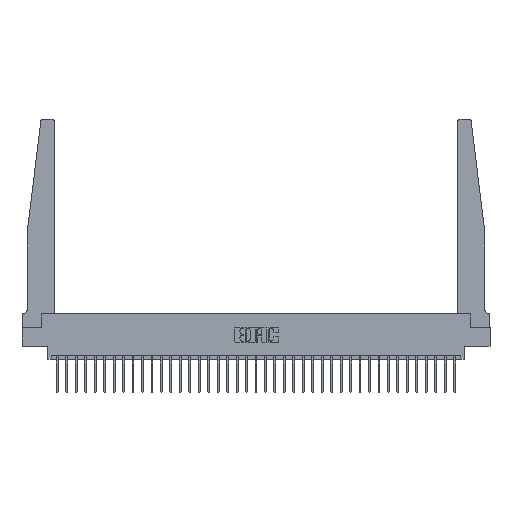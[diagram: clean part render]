
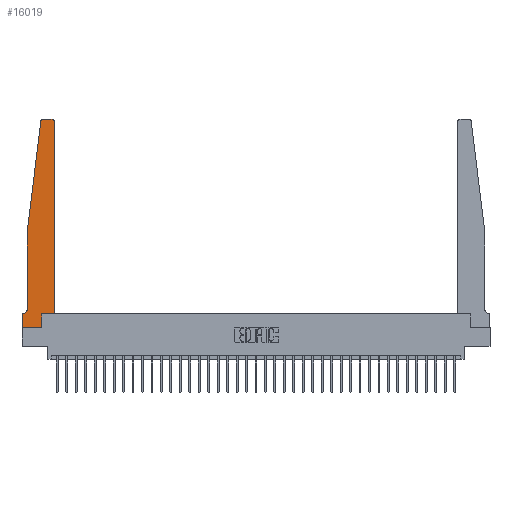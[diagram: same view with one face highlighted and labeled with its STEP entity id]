
A CAD part, top view. The second image highlights one B-rep face of the part: STEP entity #16019.
In plain terms, the highlighted planar face has unit normal (0, 0, 1).
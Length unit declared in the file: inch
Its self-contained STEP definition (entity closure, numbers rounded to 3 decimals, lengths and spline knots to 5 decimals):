
#213 = VECTOR ( 'NONE', #19562, 39.37008 ) ;
#295 = AXIS2_PLACEMENT_3D ( 'NONE', #20540, #5225, #23086 ) ;
#1039 = ORIENTED_EDGE ( 'NONE', *, *, #8763, .T. ) ;
#1201 = DIRECTION ( 'NONE',  ( -1., 0., 0. ) ) ;
#1218 = CARTESIAN_POINT ( 'NONE',  ( 0.065, 1.25, 0.37 ) ) ;
#1359 = CARTESIAN_POINT ( 'NONE',  ( 0., 0., 0.37 ) ) ;
#1548 = VERTEX_POINT ( 'NONE', #15103 ) ;
#1581 = ORIENTED_EDGE ( 'NONE', *, *, #18821, .T. ) ;
#1651 = CARTESIAN_POINT ( 'NONE',  ( 0.2605, 0.18, 0.37 ) ) ;
#1680 = VERTEX_POINT ( 'NONE', #15545 ) ;
#1836 = DIRECTION ( 'NONE',  ( 1., 0., 0. ) ) ;
#2565 = VERTEX_POINT ( 'NONE', #21839 ) ;
#2676 = LINE ( 'NONE', #16550, #31295 ) ;
#3178 = EDGE_CURVE ( 'NONE', #5346, #8923, #9283, .T. ) ;
#4044 = CARTESIAN_POINT ( 'NONE',  ( 0., 0., 0.37 ) ) ;
#4154 = DIRECTION ( 'NONE',  ( 0., -1., 0. ) ) ;
#4301 = CIRCLE ( 'NONE', #295, 0.05 ) ;
#4777 = DIRECTION ( 'NONE',  ( 0., -1., 0. ) ) ;
#4904 = AXIS2_PLACEMENT_3D ( 'NONE', #11142, #28911, #13719 ) ;
#5198 = LINE ( 'NONE', #8431, #18011 ) ;
#5225 = DIRECTION ( 'NONE',  ( 0., 0., -1. ) ) ;
#5346 = VERTEX_POINT ( 'NONE', #24933 ) ;
#5541 = CARTESIAN_POINT ( 'NONE',  ( 0.27653, 2.72, 0.37 ) ) ;
#5909 = CARTESIAN_POINT ( 'NONE',  ( 0.395, 2.72, 0.37 ) ) ;
#5992 = PLANE ( 'NONE',  #4904 ) ;
#6184 = EDGE_CURVE ( 'NONE', #6297, #2565, #2676, .T. ) ;
#6297 = VERTEX_POINT ( 'NONE', #26972 ) ;
#6372 = ORIENTED_EDGE ( 'NONE', *, *, #26674, .T. ) ;
#6871 = CARTESIAN_POINT ( 'NONE',  ( 0.425, 0.18, 0.37 ) ) ;
#7365 = LINE ( 'NONE', #25215, #20162 ) ;
#7714 = EDGE_CURVE ( 'NONE', #30909, #18710, #8582, .T. ) ;
#8124 = DIRECTION ( 'NONE',  ( 1., 0., 0. ) ) ;
#8431 = CARTESIAN_POINT ( 'NONE',  ( 0.065, 0.1875, 0.37 ) ) ;
#8477 = DIRECTION ( 'NONE',  ( 1., 0., 0. ) ) ;
#8582 = LINE ( 'NONE', #22020, #28882 ) ;
#8763 = EDGE_CURVE ( 'NONE', #2565, #27652, #12119, .T. ) ;
#8913 = EDGE_LOOP ( 'NONE', ( #11720, #1039, #6372, #1581, #9547, #12216, #17076, #16816, #17228, #18980, #19419, #20133 ) ) ;
#8923 = VERTEX_POINT ( 'NONE', #1359 ) ;
#9283 = LINE ( 'NONE', #4044, #28784 ) ;
#9547 = ORIENTED_EDGE ( 'NONE', *, *, #22452, .T. ) ;
#10999 = AXIS2_PLACEMENT_3D ( 'NONE', #5541, #23408, #8124 ) ;
#11142 = CARTESIAN_POINT ( 'NONE',  ( 0., 0.1875, 0.37 ) ) ;
#11720 = ORIENTED_EDGE ( 'NONE', *, *, #6184, .T. ) ;
#11941 = CARTESIAN_POINT ( 'NONE',  ( 0.425, 0.18, 0.37 ) ) ;
#12119 = CIRCLE ( 'NONE', #10999, 0.03 ) ;
#12216 = ORIENTED_EDGE ( 'NONE', *, *, #26487, .T. ) ;
#13167 = EDGE_CURVE ( 'NONE', #8923, #23413, #18066, .T. ) ;
#13215 = LINE ( 'NONE', #32011, #19977 ) ;
#13719 = DIRECTION ( 'NONE',  ( 1., 0., 0. ) ) ;
#14619 = CARTESIAN_POINT ( 'NONE',  ( 0., 0., 0.37 ) ) ;
#15103 = CARTESIAN_POINT ( 'NONE',  ( 0.065, 0.2375, 0.37 ) ) ;
#15545 = CARTESIAN_POINT ( 'NONE',  ( 0.425, 2.72, 0.37 ) ) ;
#16019 = ADVANCED_FACE ( 'NONE', ( #17477 ), #5992, .T. ) ;
#16267 = EDGE_CURVE ( 'NONE', #18710, #1680, #23837, .T. ) ;
#16524 = CARTESIAN_POINT ( 'NONE',  ( 0.2605, 0.18, 0.37 ) ) ;
#16550 = CARTESIAN_POINT ( 'NONE',  ( 0.25, 2.75, 0.37 ) ) ;
#16816 = ORIENTED_EDGE ( 'NONE', *, *, #13167, .T. ) ;
#16880 = EDGE_CURVE ( 'NONE', #23413, #30909, #19827, .T. ) ;
#16916 = DIRECTION ( 'NONE',  ( -0.122, -0.992, 0. ) ) ;
#17058 = VECTOR ( 'NONE', #32218, 39.37008 ) ;
#17076 = ORIENTED_EDGE ( 'NONE', *, *, #3178, .T. ) ;
#17228 = ORIENTED_EDGE ( 'NONE', *, *, #16880, .T. ) ;
#17328 = EDGE_CURVE ( 'NONE', #1680, #6297, #28116, .T. ) ;
#17477 = FACE_OUTER_BOUND ( 'NONE', #8913, .T. ) ;
#18011 = VECTOR ( 'NONE', #31153, 39.37008 ) ;
#18066 = LINE ( 'NONE', #14619, #23231 ) ;
#18710 = VERTEX_POINT ( 'NONE', #11941 ) ;
#18821 = EDGE_CURVE ( 'NONE', #19816, #1548, #7365, .T. ) ;
#18980 = ORIENTED_EDGE ( 'NONE', *, *, #7714, .T. ) ;
#19419 = ORIENTED_EDGE ( 'NONE', *, *, #16267, .T. ) ;
#19562 = DIRECTION ( 'NONE',  ( 0., 1., 0. ) ) ;
#19816 = VERTEX_POINT ( 'NONE', #1218 ) ;
#19827 = LINE ( 'NONE', #1651, #213 ) ;
#19977 = VECTOR ( 'NONE', #16916, 39.37008 ) ;
#20133 = ORIENTED_EDGE ( 'NONE', *, *, #17328, .T. ) ;
#20162 = VECTOR ( 'NONE', #4777, 39.37008 ) ;
#20540 = CARTESIAN_POINT ( 'NONE',  ( 0.015, 0.2375, 0.37 ) ) ;
#21839 = CARTESIAN_POINT ( 'NONE',  ( 0.27653, 2.75, 0.37 ) ) ;
#22020 = CARTESIAN_POINT ( 'NONE',  ( 0.425, 0.18, 0.37 ) ) ;
#22452 = EDGE_CURVE ( 'NONE', #1548, #24305, #4301, .T. ) ;
#23086 = DIRECTION ( 'NONE',  ( -1., 0., 0. ) ) ;
#23231 = VECTOR ( 'NONE', #1836, 39.37008 ) ;
#23408 = DIRECTION ( 'NONE',  ( 0., 0., 1. ) ) ;
#23413 = VERTEX_POINT ( 'NONE', #24577 ) ;
#23766 = DIRECTION ( 'NONE',  ( 0., 0., 1. ) ) ;
#23837 = LINE ( 'NONE', #6871, #17058 ) ;
#24289 = CARTESIAN_POINT ( 'NONE',  ( 0.015, 0.1875, 0.37 ) ) ;
#24305 = VERTEX_POINT ( 'NONE', #24289 ) ;
#24577 = CARTESIAN_POINT ( 'NONE',  ( 0.2605, 0., 0.37 ) ) ;
#24589 = DIRECTION ( 'NONE',  ( 1., 0., 0. ) ) ;
#24933 = CARTESIAN_POINT ( 'NONE',  ( 0., 0.1875, 0.37 ) ) ;
#25215 = CARTESIAN_POINT ( 'NONE',  ( 0.065, 1.25, 0.37 ) ) ;
#26487 = EDGE_CURVE ( 'NONE', #24305, #5346, #5198, .T. ) ;
#26674 = EDGE_CURVE ( 'NONE', #27652, #19816, #13215, .T. ) ;
#26751 = CARTESIAN_POINT ( 'NONE',  ( 0.24675, 2.72367, 0.37 ) ) ;
#26972 = CARTESIAN_POINT ( 'NONE',  ( 0.395, 2.75, 0.37 ) ) ;
#27652 = VERTEX_POINT ( 'NONE', #26751 ) ;
#28116 = CIRCLE ( 'NONE', #28612, 0.03 ) ;
#28612 = AXIS2_PLACEMENT_3D ( 'NONE', #5909, #23766, #8477 ) ;
#28784 = VECTOR ( 'NONE', #4154, 39.37008 ) ;
#28882 = VECTOR ( 'NONE', #24589, 39.37008 ) ;
#28911 = DIRECTION ( 'NONE',  ( 0., 0., 1. ) ) ;
#30909 = VERTEX_POINT ( 'NONE', #16524 ) ;
#31153 = DIRECTION ( 'NONE',  ( -1., 0., 0. ) ) ;
#31295 = VECTOR ( 'NONE', #1201, 39.37008 ) ;
#32011 = CARTESIAN_POINT ( 'NONE',  ( 0.065, 1.25, 0.37 ) ) ;
#32218 = DIRECTION ( 'NONE',  ( 0., 1., 0. ) ) ;
